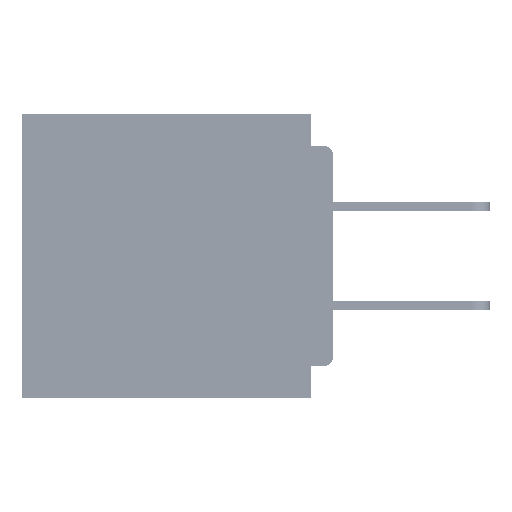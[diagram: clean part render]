
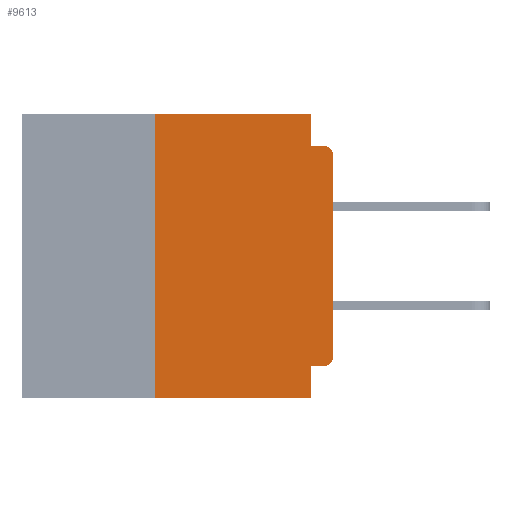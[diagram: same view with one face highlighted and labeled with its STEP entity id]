
A CAD part, left-side view. The second image highlights one B-rep face of the part: STEP entity #9613.
In plain terms, the highlighted planar face has unit normal (-1, 0, 0).
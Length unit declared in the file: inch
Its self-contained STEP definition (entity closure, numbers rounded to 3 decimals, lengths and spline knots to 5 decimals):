
#604 = CARTESIAN_POINT ( 'NONE',  ( 0., 0.25, -0.4 ) ) ;
#967 = VECTOR ( 'NONE', #17095, 39.37008 ) ;
#1050 = VECTOR ( 'NONE', #61448, 39.37008 ) ;
#1466 = ORIENTED_EDGE ( 'NONE', *, *, #11192, .F. ) ;
#1806 = CIRCLE ( 'NONE', #15459, 0.015 ) ;
#1820 = LINE ( 'NONE', #29207, #48067 ) ;
#2543 = LINE ( 'NONE', #18511, #1050 ) ;
#2868 = DIRECTION ( 'NONE',  ( -1., 0., 0. ) ) ;
#3016 = LINE ( 'NONE', #31151, #26883 ) ;
#3344 = VERTEX_POINT ( 'NONE', #49219 ) ;
#3835 = DIRECTION ( 'NONE',  ( -1., 0., 0. ) ) ;
#5461 = DIRECTION ( 'NONE',  ( 0., 1., 0. ) ) ;
#6063 = CIRCLE ( 'NONE', #48671, 0.015 ) ;
#7343 = VERTEX_POINT ( 'NONE', #54201 ) ;
#8176 = CARTESIAN_POINT ( 'NONE',  ( 0., 0.031, -0.355 ) ) ;
#8248 = VERTEX_POINT ( 'NONE', #18422 ) ;
#8426 = EDGE_CURVE ( 'NONE', #56953, #8248, #30595, .T. ) ;
#9613 = ADVANCED_FACE ( 'NONE', ( #36349 ), #23527, .F. ) ;
#9720 = VERTEX_POINT ( 'NONE', #604 ) ;
#11192 = EDGE_CURVE ( 'NONE', #22145, #25341, #56325, .T. ) ;
#11431 = CARTESIAN_POINT ( 'NONE',  ( 0., 0.437, -0.4 ) ) ;
#12013 = EDGE_CURVE ( 'NONE', #54349, #56953, #1806, .T. ) ;
#12764 = CARTESIAN_POINT ( 'NONE',  ( 0., 0., -0.34 ) ) ;
#13561 = EDGE_LOOP ( 'NONE', ( #15530, #19210, #1466, #24012, #38966, #31396, #19070, #37037, #34241, #22210 ) ) ;
#15201 = VECTOR ( 'NONE', #16169, 39.37008 ) ;
#15459 = AXIS2_PLACEMENT_3D ( 'NONE', #32347, #3835, #37119 ) ;
#15530 = ORIENTED_EDGE ( 'NONE', *, *, #8426, .T. ) ;
#16169 = DIRECTION ( 'NONE',  ( 0., -1., 0. ) ) ;
#16914 = VERTEX_POINT ( 'NONE', #8176 ) ;
#17095 = DIRECTION ( 'NONE',  ( 0., -1., 0. ) ) ;
#17180 = CARTESIAN_POINT ( 'NONE',  ( 0., 0.031, -0.4 ) ) ;
#18422 = CARTESIAN_POINT ( 'NONE',  ( 0., 0., -0.06 ) ) ;
#18511 = CARTESIAN_POINT ( 'NONE',  ( 0., 0.031, 0. ) ) ;
#19070 = ORIENTED_EDGE ( 'NONE', *, *, #36505, .T. ) ;
#19210 = ORIENTED_EDGE ( 'NONE', *, *, #22316, .T. ) ;
#19466 = CARTESIAN_POINT ( 'NONE',  ( 0., 0., 0. ) ) ;
#21586 = DIRECTION ( 'NONE',  ( 0., 0., 1. ) ) ;
#22145 = VERTEX_POINT ( 'NONE', #39749 ) ;
#22210 = ORIENTED_EDGE ( 'NONE', *, *, #12013, .T. ) ;
#22316 = EDGE_CURVE ( 'NONE', #8248, #25341, #6063, .T. ) ;
#23527 = PLANE ( 'NONE',  #31335 ) ;
#24012 = ORIENTED_EDGE ( 'NONE', *, *, #34052, .F. ) ;
#24778 = CARTESIAN_POINT ( 'NONE',  ( 0., 0.015, -0.355 ) ) ;
#25341 = VERTEX_POINT ( 'NONE', #57104 ) ;
#26883 = VECTOR ( 'NONE', #21586, 39.37008 ) ;
#27747 = VECTOR ( 'NONE', #55389, 39.37008 ) ;
#27819 = LINE ( 'NONE', #31287, #967 ) ;
#28320 = CARTESIAN_POINT ( 'NONE',  ( 0., 0.437, 0. ) ) ;
#29124 = VECTOR ( 'NONE', #33834, 39.37008 ) ;
#29207 = CARTESIAN_POINT ( 'NONE',  ( 0., 0., -0.355 ) ) ;
#30595 = LINE ( 'NONE', #19466, #29124 ) ;
#31151 = CARTESIAN_POINT ( 'NONE',  ( 0., 0.25, -0.4 ) ) ;
#31287 = CARTESIAN_POINT ( 'NONE',  ( 0., 0.437, 0. ) ) ;
#31335 = AXIS2_PLACEMENT_3D ( 'NONE', #28320, #61613, #33086 ) ;
#31377 = CARTESIAN_POINT ( 'NONE',  ( 0., 0.015, -0.06 ) ) ;
#31396 = ORIENTED_EDGE ( 'NONE', *, *, #50016, .F. ) ;
#32347 = CARTESIAN_POINT ( 'NONE',  ( 0., 0.015, -0.34 ) ) ;
#33086 = DIRECTION ( 'NONE',  ( 0., 0., -1. ) ) ;
#33834 = DIRECTION ( 'NONE',  ( 0., 0., 1. ) ) ;
#34052 = EDGE_CURVE ( 'NONE', #7343, #22145, #2543, .T. ) ;
#34241 = ORIENTED_EDGE ( 'NONE', *, *, #61083, .F. ) ;
#36146 = DIRECTION ( 'NONE',  ( 0., 0., -1. ) ) ;
#36349 = FACE_OUTER_BOUND ( 'NONE', #13561, .T. ) ;
#36505 = EDGE_CURVE ( 'NONE', #9720, #39077, #53280, .T. ) ;
#37037 = ORIENTED_EDGE ( 'NONE', *, *, #43249, .F. ) ;
#37119 = DIRECTION ( 'NONE',  ( 0., 0., -1. ) ) ;
#38966 = ORIENTED_EDGE ( 'NONE', *, *, #55088, .F. ) ;
#39077 = VERTEX_POINT ( 'NONE', #39098 ) ;
#39098 = CARTESIAN_POINT ( 'NONE',  ( 0., 0.031, -0.4 ) ) ;
#39749 = CARTESIAN_POINT ( 'NONE',  ( 0., 0.031, -0.045 ) ) ;
#43249 = EDGE_CURVE ( 'NONE', #16914, #39077, #54605, .T. ) ;
#43655 = VECTOR ( 'NONE', #45184, 39.37008 ) ;
#45184 = DIRECTION ( 'NONE',  ( 0., -1., 0. ) ) ;
#48067 = VECTOR ( 'NONE', #5461, 39.37008 ) ;
#48671 = AXIS2_PLACEMENT_3D ( 'NONE', #31377, #2868, #36146 ) ;
#49219 = CARTESIAN_POINT ( 'NONE',  ( 0., 0.25, 0. ) ) ;
#50016 = EDGE_CURVE ( 'NONE', #9720, #3344, #3016, .T. ) ;
#53280 = LINE ( 'NONE', #11431, #15201 ) ;
#54201 = CARTESIAN_POINT ( 'NONE',  ( 0., 0.031, 0. ) ) ;
#54349 = VERTEX_POINT ( 'NONE', #24778 ) ;
#54605 = LINE ( 'NONE', #17180, #27747 ) ;
#55088 = EDGE_CURVE ( 'NONE', #3344, #7343, #27819, .T. ) ;
#55389 = DIRECTION ( 'NONE',  ( 0., 0., -1. ) ) ;
#56325 = LINE ( 'NONE', #59311, #43655 ) ;
#56953 = VERTEX_POINT ( 'NONE', #12764 ) ;
#57104 = CARTESIAN_POINT ( 'NONE',  ( 0., 0.015, -0.045 ) ) ;
#59311 = CARTESIAN_POINT ( 'NONE',  ( 0., 0., -0.045 ) ) ;
#61083 = EDGE_CURVE ( 'NONE', #54349, #16914, #1820, .T. ) ;
#61448 = DIRECTION ( 'NONE',  ( 0., 0., -1. ) ) ;
#61613 = DIRECTION ( 'NONE',  ( 1., 0., 0. ) ) ;
